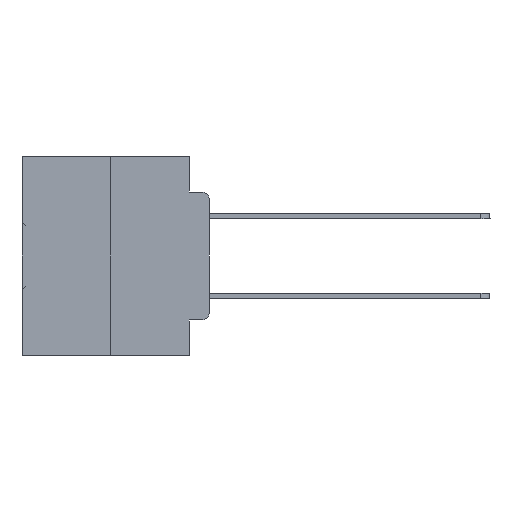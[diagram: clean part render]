
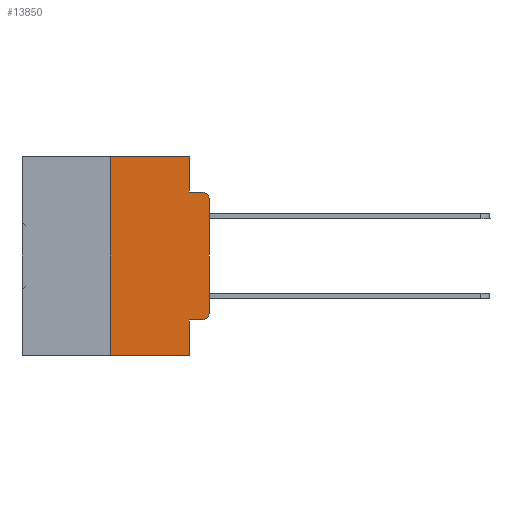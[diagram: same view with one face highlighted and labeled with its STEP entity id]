
A CAD part, left-side view. The second image highlights one B-rep face of the part: STEP entity #13850.
In plain terms, the highlighted planar face has unit normal (-1, 0, 0).
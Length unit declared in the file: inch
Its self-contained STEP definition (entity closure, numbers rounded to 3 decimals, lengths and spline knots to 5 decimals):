
#1413 = FACE_OUTER_BOUND ( 'NONE', #36532, .T. ) ;
#1708 = DIRECTION ( 'NONE',  ( 0., -1., 0. ) ) ;
#1780 = CARTESIAN_POINT ( 'NONE',  ( 0., 0., -0.3915 ) ) ;
#2153 = VECTOR ( 'NONE', #6608, 39.37008 ) ;
#2442 = AXIS2_PLACEMENT_3D ( 'NONE', #27647, #12904, #9900 ) ;
#2816 = DIRECTION ( 'NONE',  ( 0., 0., 1. ) ) ;
#2893 = CARTESIAN_POINT ( 'NONE',  ( 0., 0.02, -0.3915 ) ) ;
#3099 = VERTEX_POINT ( 'NONE', #7258 ) ;
#3224 = CARTESIAN_POINT ( 'NONE',  ( 0., 0.051, -0.0885 ) ) ;
#3808 = EDGE_CURVE ( 'NONE', #22015, #21653, #29831, .T. ) ;
#4938 = VECTOR ( 'NONE', #8973, 39.37008 ) ;
#5141 = LINE ( 'NONE', #19861, #32544 ) ;
#5550 = DIRECTION ( 'NONE',  ( 0., 0., -1. ) ) ;
#5808 = EDGE_CURVE ( 'NONE', #9050, #6974, #34131, .T. ) ;
#5868 = VECTOR ( 'NONE', #6255, 39.37008 ) ;
#6255 = DIRECTION ( 'NONE',  ( 0., -1., 0. ) ) ;
#6608 = DIRECTION ( 'NONE',  ( 0., -1., 0. ) ) ;
#6728 = DIRECTION ( 'NONE',  ( 0., -1., 0. ) ) ;
#6974 = VERTEX_POINT ( 'NONE', #1780 ) ;
#7258 = CARTESIAN_POINT ( 'NONE',  ( 0., 0., -0.1085 ) ) ;
#7260 = AXIS2_PLACEMENT_3D ( 'NONE', #11057, #25785, #20124 ) ;
#7587 = EDGE_CURVE ( 'NONE', #22015, #21524, #5141, .T. ) ;
#7863 = CARTESIAN_POINT ( 'NONE',  ( 0., 0.02, -0.0885 ) ) ;
#8176 = CARTESIAN_POINT ( 'NONE',  ( 0., 0.051, -0.5 ) ) ;
#8972 = VERTEX_POINT ( 'NONE', #17009 ) ;
#8973 = DIRECTION ( 'NONE',  ( 0., 0., -1. ) ) ;
#9050 = VERTEX_POINT ( 'NONE', #20975 ) ;
#9049 = EDGE_CURVE ( 'NONE', #34087, #15366, #17562, .T. ) ;
#9900 = DIRECTION ( 'NONE',  ( 0., 0., -1. ) ) ;
#10817 = DIRECTION ( 'NONE',  ( -1., 0., 0. ) ) ;
#11034 = VECTOR ( 'NONE', #6728, 39.37008 ) ;
#11057 = CARTESIAN_POINT ( 'NONE',  ( 0., 0.02, -0.1085 ) ) ;
#11862 = LINE ( 'NONE', #29060, #17114 ) ;
#12644 = CARTESIAN_POINT ( 'NONE',  ( 0., 0.051, -0.4115 ) ) ;
#12904 = DIRECTION ( 'NONE',  ( 1., 0., 0. ) ) ;
#13169 = ORIENTED_EDGE ( 'NONE', *, *, #22389, .F. ) ;
#13602 = DIRECTION ( 'NONE',  ( 0., 0., 1. ) ) ;
#13850 = ADVANCED_FACE ( 'NONE', ( #1413 ), #32786, .F. ) ;
#15079 = ORIENTED_EDGE ( 'NONE', *, *, #37209, .T. ) ;
#15181 = EDGE_CURVE ( 'NONE', #6974, #3099, #11862, .T. ) ;
#15366 = VERTEX_POINT ( 'NONE', #7863 ) ;
#15756 = LINE ( 'NONE', #24642, #11034 ) ;
#16349 = CARTESIAN_POINT ( 'NONE',  ( 0., 0.051, 0. ) ) ;
#16695 = ORIENTED_EDGE ( 'NONE', *, *, #22671, .F. ) ;
#17009 = CARTESIAN_POINT ( 'NONE',  ( 0., 0.051, 0. ) ) ;
#17114 = VECTOR ( 'NONE', #2816, 39.37008 ) ;
#17562 = LINE ( 'NONE', #3224, #5868 ) ;
#17730 = ORIENTED_EDGE ( 'NONE', *, *, #30335, .T. ) ;
#17817 = AXIS2_PLACEMENT_3D ( 'NONE', #2893, #10817, #5550 ) ;
#18831 = LINE ( 'NONE', #16349, #25994 ) ;
#19861 = CARTESIAN_POINT ( 'NONE',  ( 0., 0.25, 0. ) ) ;
#20124 = DIRECTION ( 'NONE',  ( 0., 0., -1. ) ) ;
#20975 = CARTESIAN_POINT ( 'NONE',  ( 0., 0.02, -0.4115 ) ) ;
#21524 = VERTEX_POINT ( 'NONE', #33494 ) ;
#21653 = VERTEX_POINT ( 'NONE', #8176 ) ;
#22015 = VERTEX_POINT ( 'NONE', #30605 ) ;
#22389 = EDGE_CURVE ( 'NONE', #27778, #21653, #18831, .T. ) ;
#22671 = EDGE_CURVE ( 'NONE', #8972, #34087, #32236, .T. ) ;
#23150 = CARTESIAN_POINT ( 'NONE',  ( 0., 0.051, 0. ) ) ;
#23829 = ORIENTED_EDGE ( 'NONE', *, *, #5808, .T. ) ;
#24002 = LINE ( 'NONE', #12644, #26781 ) ;
#24642 = CARTESIAN_POINT ( 'NONE',  ( 0., 0.473, 0. ) ) ;
#24935 = ORIENTED_EDGE ( 'NONE', *, *, #7587, .F. ) ;
#25638 = ORIENTED_EDGE ( 'NONE', *, *, #9049, .F. ) ;
#25785 = DIRECTION ( 'NONE',  ( -1., 0., 0. ) ) ;
#25994 = VECTOR ( 'NONE', #33393, 39.37008 ) ;
#26233 = CARTESIAN_POINT ( 'NONE',  ( 0., 0.473, -0.5 ) ) ;
#26781 = VECTOR ( 'NONE', #1708, 39.37008 ) ;
#27647 = CARTESIAN_POINT ( 'NONE',  ( 0., 0.473, 0. ) ) ;
#27762 = CIRCLE ( 'NONE', #7260, 0.02 ) ;
#27778 = VERTEX_POINT ( 'NONE', #29306 ) ;
#29060 = CARTESIAN_POINT ( 'NONE',  ( 0., 0., 0. ) ) ;
#29306 = CARTESIAN_POINT ( 'NONE',  ( 0., 0.051, -0.4115 ) ) ;
#29831 = LINE ( 'NONE', #26233, #2153 ) ;
#29972 = ORIENTED_EDGE ( 'NONE', *, *, #3808, .T. ) ;
#30145 = ORIENTED_EDGE ( 'NONE', *, *, #34941, .F. ) ;
#30335 = EDGE_CURVE ( 'NONE', #3099, #15366, #27762, .T. ) ;
#30605 = CARTESIAN_POINT ( 'NONE',  ( 0., 0.25, -0.5 ) ) ;
#32236 = LINE ( 'NONE', #23150, #4938 ) ;
#32544 = VECTOR ( 'NONE', #13602, 39.37008 ) ;
#32786 = PLANE ( 'NONE',  #2442 ) ;
#33393 = DIRECTION ( 'NONE',  ( 0., 0., -1. ) ) ;
#33494 = CARTESIAN_POINT ( 'NONE',  ( 0., 0.25, 0. ) ) ;
#34087 = VERTEX_POINT ( 'NONE', #36908 ) ;
#34131 = CIRCLE ( 'NONE', #17817, 0.02 ) ;
#34941 = EDGE_CURVE ( 'NONE', #21524, #8972, #15756, .T. ) ;
#36207 = ORIENTED_EDGE ( 'NONE', *, *, #15181, .T. ) ;
#36532 = EDGE_LOOP ( 'NONE', ( #36207, #17730, #25638, #16695, #30145, #24935, #29972, #13169, #15079, #23829 ) ) ;
#36908 = CARTESIAN_POINT ( 'NONE',  ( 0., 0.051, -0.0885 ) ) ;
#37209 = EDGE_CURVE ( 'NONE', #27778, #9050, #24002, .T. ) ;
